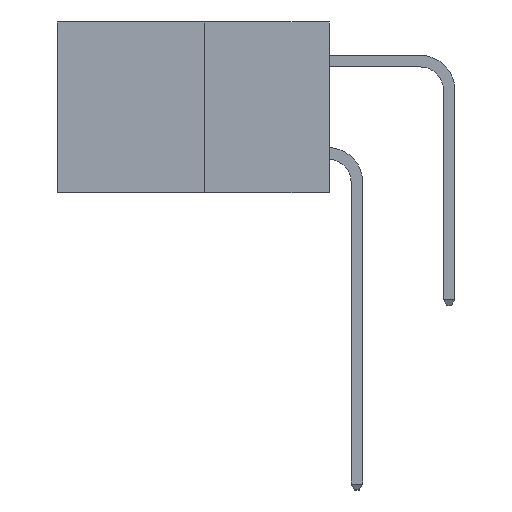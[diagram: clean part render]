
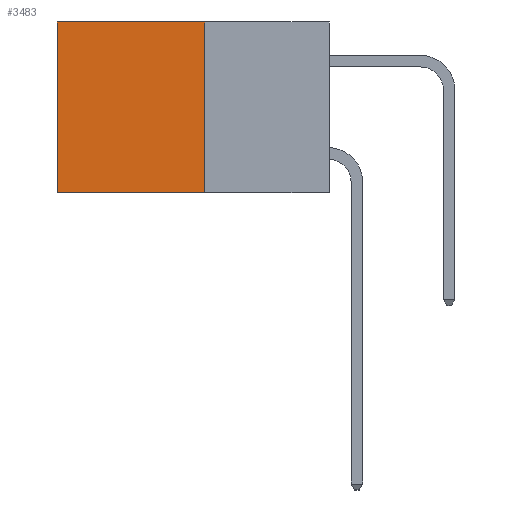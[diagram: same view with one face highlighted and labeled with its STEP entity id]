
A CAD part, left-side view. The second image highlights one B-rep face of the part: STEP entity #3483.
In plain terms, the highlighted planar face has unit normal (-1, 0, 0).
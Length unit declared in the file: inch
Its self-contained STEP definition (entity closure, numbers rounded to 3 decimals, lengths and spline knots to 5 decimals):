
#221 = DIRECTION ( 'NONE',  ( 0., 0., -1. ) ) ;
#297 = ORIENTED_EDGE ( 'NONE', *, *, #5110, .T. ) ;
#323 = DIRECTION ( 'NONE',  ( 1., 0., 0. ) ) ;
#342 = CARTESIAN_POINT ( 'NONE',  ( 0.277, 0.27, -0.37 ) ) ;
#508 = EDGE_CURVE ( 'NONE', #4613, #12646, #16509, .T. ) ;
#557 = PLANE ( 'NONE',  #14766 ) ;
#1842 = CARTESIAN_POINT ( 'NONE',  ( 0.277, 0.27, 0. ) ) ;
#2615 = CARTESIAN_POINT ( 'NONE',  ( 0.277, 0.27, -0.37 ) ) ;
#2778 = CARTESIAN_POINT ( 'NONE',  ( 0.277, 0.59, 0. ) ) ;
#2824 = DIRECTION ( 'NONE',  ( 0., 0., -1. ) ) ;
#3483 = ADVANCED_FACE ( 'NONE', ( #12952 ), #557, .F. ) ;
#4168 = ORIENTED_EDGE ( 'NONE', *, *, #508, .F. ) ;
#4291 = DIRECTION ( 'NONE',  ( 0., 1., 0. ) ) ;
#4613 = VERTEX_POINT ( 'NONE', #1842 ) ;
#4882 = VECTOR ( 'NONE', #2824, 39.37008 ) ;
#5110 = EDGE_CURVE ( 'NONE', #10872, #13619, #6349, .T. ) ;
#6349 = LINE ( 'NONE', #16440, #15557 ) ;
#7091 = LINE ( 'NONE', #14941, #16603 ) ;
#8500 = CARTESIAN_POINT ( 'NONE',  ( 0.277, 0.27, -0.37 ) ) ;
#8800 = DIRECTION ( 'NONE',  ( 0., 0., -1. ) ) ;
#9712 = CARTESIAN_POINT ( 'NONE',  ( 0.277, 0.27, 0. ) ) ;
#9878 = DIRECTION ( 'NONE',  ( 0., 1., 0. ) ) ;
#10031 = LINE ( 'NONE', #9712, #13076 ) ;
#10305 = EDGE_CURVE ( 'NONE', #4613, #10872, #10031, .T. ) ;
#10872 = VERTEX_POINT ( 'NONE', #2778 ) ;
#11000 = EDGE_LOOP ( 'NONE', ( #297, #13273, #4168, #15296 ) ) ;
#12646 = VERTEX_POINT ( 'NONE', #8500 ) ;
#12952 = FACE_OUTER_BOUND ( 'NONE', #11000, .T. ) ;
#13076 = VECTOR ( 'NONE', #4291, 39.37008 ) ;
#13273 = ORIENTED_EDGE ( 'NONE', *, *, #13861, .F. ) ;
#13301 = CARTESIAN_POINT ( 'NONE',  ( 0.277, 0.59, -0.37 ) ) ;
#13619 = VERTEX_POINT ( 'NONE', #13301 ) ;
#13861 = EDGE_CURVE ( 'NONE', #12646, #13619, #7091, .T. ) ;
#14766 = AXIS2_PLACEMENT_3D ( 'NONE', #342, #323, #221 ) ;
#14941 = CARTESIAN_POINT ( 'NONE',  ( 0.277, 0.27, -0.37 ) ) ;
#15296 = ORIENTED_EDGE ( 'NONE', *, *, #10305, .T. ) ;
#15557 = VECTOR ( 'NONE', #8800, 39.37008 ) ;
#16440 = CARTESIAN_POINT ( 'NONE',  ( 0.277, 0.59, -0.37 ) ) ;
#16509 = LINE ( 'NONE', #2615, #4882 ) ;
#16603 = VECTOR ( 'NONE', #9878, 39.37008 ) ;
